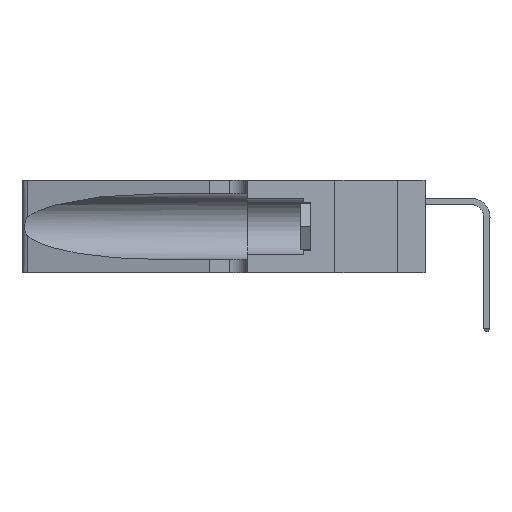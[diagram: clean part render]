
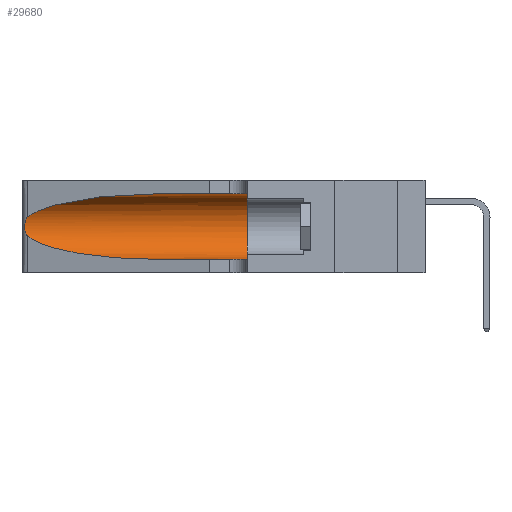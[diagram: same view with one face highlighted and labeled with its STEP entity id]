
A CAD part, left-side view. The second image highlights one B-rep face of the part: STEP entity #29680.
In plain terms, the highlighted cylindrical face has radius 3.308 mm (diameter 6.617 mm), a partial arc.
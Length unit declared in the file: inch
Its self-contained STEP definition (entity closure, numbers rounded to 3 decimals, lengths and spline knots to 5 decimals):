
#218 =( BOUNDED_CURVE ( )  B_SPLINE_CURVE ( 3, ( #10784, #19612, #1523, #22807 ),
 .UNSPECIFIED., .F., .T. ) 
 B_SPLINE_CURVE_WITH_KNOTS ( ( 4, 4 ),
 ( 1.5708, 2.84003 ),
 .UNSPECIFIED. ) 
 CURVE ( )  GEOMETRIC_REPRESENTATION_ITEM ( )  RATIONAL_B_SPLINE_CURVE ( ( 1., 0.87, 0.87, 1. ) ) 
 REPRESENTATION_ITEM ( '' )  );
#262 = ORIENTED_EDGE ( 'NONE', *, *, #8094, .T. ) ;
#878 = EDGE_LOOP ( 'NONE', ( #12687, #28613, #13674, #262, #2184, #4011 ) ) ;
#1523 = CARTESIAN_POINT ( 'NONE',  ( 0.2373, 1.15595, 0.28018 ) ) ;
#2184 = ORIENTED_EDGE ( 'NONE', *, *, #10710, .F. ) ;
#2189 = VECTOR ( 'NONE', #13675, 39.37008 ) ;
#2564 = VERTEX_POINT ( 'NONE', #10415 ) ;
#2628 = CARTESIAN_POINT ( 'NONE',  ( 0.25789, 1.23486, 0.15765 ) ) ;
#3575 = DIRECTION ( 'NONE',  ( 0., -1., 0. ) ) ;
#4011 = ORIENTED_EDGE ( 'NONE', *, *, #36444, .F. ) ;
#4753 = CARTESIAN_POINT ( 'NONE',  ( 0.25487, 1.22718, 0.14631 ) ) ;
#5473 = CARTESIAN_POINT ( 'NONE',  ( 0.1305, 1.61858, 0.185 ) ) ;
#5621 = CARTESIAN_POINT ( 'NONE',  ( 0.25555, 1.22994, 0.2215 ) ) ;
#5754 = CARTESIAN_POINT ( 'NONE',  ( 0.25555, 1.22993, 0.14849 ) ) ;
#6615 = CARTESIAN_POINT ( 'NONE',  ( 0.1305, 0.35, 0.05475 ) ) ;
#7263 = VERTEX_POINT ( 'NONE', #27429 ) ;
#7668 = CARTESIAN_POINT ( 'NONE',  ( 0.25487, 1.22718, 0.14631 ) ) ;
#8094 = EDGE_CURVE ( 'NONE', #2564, #22523, #10480, .T. ) ;
#8436 = CARTESIAN_POINT ( 'NONE',  ( 0.1305, 0.35, 0.31525 ) ) ;
#8622 = CARTESIAN_POINT ( 'NONE',  ( 0.25487, 1.22718, 0.22369 ) ) ;
#9001 = VERTEX_POINT ( 'NONE', #8436 ) ;
#10028 = CYLINDRICAL_SURFACE ( 'NONE', #26446, 0.13025 ) ;
#10207 = EDGE_CURVE ( 'NONE', #7263, #26656, #19950, .T. ) ;
#10415 = CARTESIAN_POINT ( 'NONE',  ( 0.1305, 0.72297, 0.05475 ) ) ;
#10480 = LINE ( 'NONE', #19650, #2189 ) ;
#10710 = EDGE_CURVE ( 'NONE', #9001, #22523, #13199, .T. ) ;
#10784 = CARTESIAN_POINT ( 'NONE',  ( 0.1305, 0.72297, 0.31525 ) ) ;
#11010 = CARTESIAN_POINT ( 'NONE',  ( 0.1305, 0.72297, 0.05475 ) ) ;
#11876 = CARTESIAN_POINT ( 'NONE',  ( 0.25787, 1.23484, 0.2124 ) ) ;
#12687 = ORIENTED_EDGE ( 'NONE', *, *, #13619, .T. ) ;
#13199 = CIRCLE ( 'NONE', #28431, 0.13025 ) ;
#13619 = EDGE_CURVE ( 'NONE', #31345, #7263, #218, .T. ) ;
#13674 = ORIENTED_EDGE ( 'NONE', *, *, #30171, .T. ) ;
#13675 = DIRECTION ( 'NONE',  ( 0., -1., 0. ) ) ;
#14931 = CARTESIAN_POINT ( 'NONE',  ( 0.26018, 1.23835, 0.19895 ) ) ;
#17510 = DIRECTION ( 'NONE',  ( 0., 1., 0. ) ) ;
#17952 = CARTESIAN_POINT ( 'NONE',  ( 0.26075, 1.23896, 0.178 ) ) ;
#19612 = CARTESIAN_POINT ( 'NONE',  ( 0.18966, 0.96281, 0.31525 ) ) ;
#19650 = CARTESIAN_POINT ( 'NONE',  ( 0.1305, 1.61858, 0.05475 ) ) ;
#19950 = B_SPLINE_CURVE_WITH_KNOTS ( 'NONE', 3,
 ( #8622, #5621, #29616, #11876, #32459, #14931, #35279, #17952, #38047, #20885, #2628, #23841, #5754, #26802 ),
 .UNSPECIFIED., .F., .F.,
 ( 4, 2, 2, 2, 2, 2, 4 ),
 ( 0., 0.00027, 0.00053, 0.00107, 0.0016, 0.00187, 0.00214 ),
 .UNSPECIFIED. ) ;
#20885 = CARTESIAN_POINT ( 'NONE',  ( 0.25856, 1.23593, 0.16098 ) ) ;
#21833 = LINE ( 'NONE', #24713, #28697 ) ;
#22523 = VERTEX_POINT ( 'NONE', #6615 ) ;
#22807 = CARTESIAN_POINT ( 'NONE',  ( 0.25487, 1.22718, 0.22369 ) ) ;
#22814 = CARTESIAN_POINT ( 'NONE',  ( 0.1305, 0.72297, 0.31525 ) ) ;
#22888 = CARTESIAN_POINT ( 'NONE',  ( 0.2373, 1.15595, 0.08982 ) ) ;
#23841 = CARTESIAN_POINT ( 'NONE',  ( 0.25639, 1.23186, 0.15144 ) ) ;
#24713 = CARTESIAN_POINT ( 'NONE',  ( 0.1305, 1.61858, 0.31525 ) ) ;
#26446 = AXIS2_PLACEMENT_3D ( 'NONE', #5473, #37916, #26530 ) ;
#26530 = DIRECTION ( 'NONE',  ( 0., 0., -1. ) ) ;
#26656 = VERTEX_POINT ( 'NONE', #7668 ) ;
#26802 = CARTESIAN_POINT ( 'NONE',  ( 0.25487, 1.22718, 0.14631 ) ) ;
#27429 = CARTESIAN_POINT ( 'NONE',  ( 0.25487, 1.22718, 0.22369 ) ) ;
#28431 = AXIS2_PLACEMENT_3D ( 'NONE', #34861, #17510, #37667 ) ;
#28613 = ORIENTED_EDGE ( 'NONE', *, *, #10207, .T. ) ;
#28697 = VECTOR ( 'NONE', #3575, 39.37008 ) ;
#28787 = CARTESIAN_POINT ( 'NONE',  ( 0.18966, 0.96281, 0.05475 ) ) ;
#29616 = CARTESIAN_POINT ( 'NONE',  ( 0.25639, 1.23184, 0.21858 ) ) ;
#29680 = ADVANCED_FACE ( 'NONE', ( #33520 ), #10028, .F. ) ;
#30171 = EDGE_CURVE ( 'NONE', #26656, #2564, #30258, .T. ) ;
#30258 =( BOUNDED_CURVE ( )  B_SPLINE_CURVE ( 3, ( #4753, #22888, #28787, #11010 ),
 .UNSPECIFIED., .F., .F. ) 
 B_SPLINE_CURVE_WITH_KNOTS ( ( 4, 4 ),
 ( 3.44316, 4.71239 ),
 .UNSPECIFIED. ) 
 CURVE ( )  GEOMETRIC_REPRESENTATION_ITEM ( )  RATIONAL_B_SPLINE_CURVE ( ( 1., 0.87, 0.87, 1. ) ) 
 REPRESENTATION_ITEM ( '' )  );
#31345 = VERTEX_POINT ( 'NONE', #22814 ) ;
#32459 = CARTESIAN_POINT ( 'NONE',  ( 0.25854, 1.2359, 0.20912 ) ) ;
#33520 = FACE_OUTER_BOUND ( 'NONE', #878, .T. ) ;
#34861 = CARTESIAN_POINT ( 'NONE',  ( 0.1305, 0.35, 0.185 ) ) ;
#35279 = CARTESIAN_POINT ( 'NONE',  ( 0.26075, 1.23896, 0.19203 ) ) ;
#36444 = EDGE_CURVE ( 'NONE', #31345, #9001, #21833, .T. ) ;
#37667 = DIRECTION ( 'NONE',  ( 0., 0., 1. ) ) ;
#37916 = DIRECTION ( 'NONE',  ( 0., -1., 0. ) ) ;
#38047 = CARTESIAN_POINT ( 'NONE',  ( 0.26017, 1.23833, 0.17102 ) ) ;
